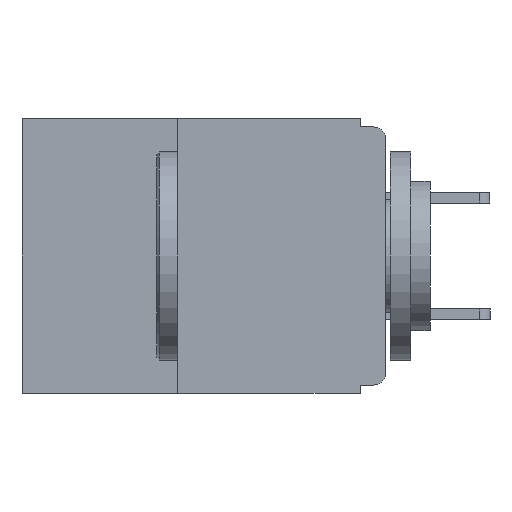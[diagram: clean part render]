
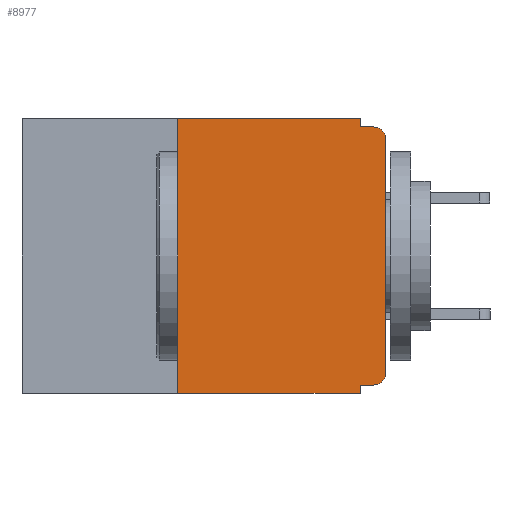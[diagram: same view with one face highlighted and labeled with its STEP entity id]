
A CAD part, left-side view. The second image highlights one B-rep face of the part: STEP entity #8977.
In plain terms, the highlighted planar face has unit normal (-1, 0, 0).
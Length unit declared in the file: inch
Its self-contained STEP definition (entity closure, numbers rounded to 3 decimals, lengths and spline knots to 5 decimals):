
#557 = VERTEX_POINT ( 'NONE', #1101 ) ;
#793 = VERTEX_POINT ( 'NONE', #4445 ) ;
#950 = VERTEX_POINT ( 'NONE', #13284 ) ;
#963 = LINE ( 'NONE', #5021, #13840 ) ;
#1101 = CARTESIAN_POINT ( 'NONE',  ( 0., 0.031, -0.01 ) ) ;
#1429 = EDGE_CURVE ( 'NONE', #14116, #10813, #10999, .T. ) ;
#1709 = ORIENTED_EDGE ( 'NONE', *, *, #15164, .F. ) ;
#1794 = ORIENTED_EDGE ( 'NONE', *, *, #3594, .F. ) ;
#1955 = CARTESIAN_POINT ( 'NONE',  ( 0., 0.015, -0.305 ) ) ;
#2170 = AXIS2_PLACEMENT_3D ( 'NONE', #1955, #12817, #3572 ) ;
#2271 = VERTEX_POINT ( 'NONE', #9158 ) ;
#2395 = ORIENTED_EDGE ( 'NONE', *, *, #1429, .T. ) ;
#2455 = ORIENTED_EDGE ( 'NONE', *, *, #19024, .F. ) ;
#2497 = ORIENTED_EDGE ( 'NONE', *, *, #18966, .F. ) ;
#3142 = LINE ( 'NONE', #9000, #7306 ) ;
#3572 = DIRECTION ( 'NONE',  ( 0., 0., -1. ) ) ;
#3594 = EDGE_CURVE ( 'NONE', #14116, #950, #7839, .T. ) ;
#3626 = CARTESIAN_POINT ( 'NONE',  ( 0., 0.031, -0.33 ) ) ;
#3959 = ORIENTED_EDGE ( 'NONE', *, *, #11931, .T. ) ;
#4445 = CARTESIAN_POINT ( 'NONE',  ( 0., 0., -0.305 ) ) ;
#5021 = CARTESIAN_POINT ( 'NONE',  ( 0., 0.031, 0. ) ) ;
#5065 = CIRCLE ( 'NONE', #2170, 0.015 ) ;
#5336 = DIRECTION ( 'NONE',  ( 0., 0., -1. ) ) ;
#5392 = EDGE_CURVE ( 'NONE', #13097, #19266, #19489, .T. ) ;
#5740 = ORIENTED_EDGE ( 'NONE', *, *, #8612, .T. ) ;
#5884 = DIRECTION ( 'NONE',  ( 0., 1., 0. ) ) ;
#5943 = AXIS2_PLACEMENT_3D ( 'NONE', #12166, #12115, #12102 ) ;
#5947 = DIRECTION ( 'NONE',  ( 0., 0., -1. ) ) ;
#6080 = CARTESIAN_POINT ( 'NONE',  ( 0., 0.25, -0.33 ) ) ;
#6108 = DIRECTION ( 'NONE',  ( 0., 0., 1. ) ) ;
#6459 = PLANE ( 'NONE',  #14403 ) ;
#6658 = VECTOR ( 'NONE', #11596, 39.37008 ) ;
#7191 = CARTESIAN_POINT ( 'NONE',  ( 0., 0.437, 0. ) ) ;
#7194 = DIRECTION ( 'NONE',  ( 0., 0., -1. ) ) ;
#7306 = VECTOR ( 'NONE', #5947, 39.37008 ) ;
#7392 = EDGE_CURVE ( 'NONE', #2271, #557, #963, .T. ) ;
#7514 = DIRECTION ( 'NONE',  ( 1., 0., 0. ) ) ;
#7839 = LINE ( 'NONE', #6080, #8315 ) ;
#8315 = VECTOR ( 'NONE', #6108, 39.37008 ) ;
#8612 = EDGE_CURVE ( 'NONE', #793, #13097, #14703, .T. ) ;
#8803 = VECTOR ( 'NONE', #18542, 39.37008 ) ;
#8830 = CARTESIAN_POINT ( 'NONE',  ( 0., 0., -0.01 ) ) ;
#8956 = VERTEX_POINT ( 'NONE', #16307 ) ;
#8977 = ADVANCED_FACE ( 'NONE', ( #19338 ), #6459, .F. ) ;
#9000 = CARTESIAN_POINT ( 'NONE',  ( 0., 0.031, -0.33 ) ) ;
#9158 = CARTESIAN_POINT ( 'NONE',  ( 0., 0.031, 0. ) ) ;
#9641 = ORIENTED_EDGE ( 'NONE', *, *, #5392, .T. ) ;
#10813 = VERTEX_POINT ( 'NONE', #3626 ) ;
#10845 = ORIENTED_EDGE ( 'NONE', *, *, #15441, .F. ) ;
#10979 = CARTESIAN_POINT ( 'NONE',  ( 0., 0.031, -0.32 ) ) ;
#10999 = LINE ( 'NONE', #18858, #11475 ) ;
#11475 = VECTOR ( 'NONE', #18968, 39.37008 ) ;
#11596 = DIRECTION ( 'NONE',  ( 0., 0., 1. ) ) ;
#11600 = CARTESIAN_POINT ( 'NONE',  ( 0., 0., 0. ) ) ;
#11920 = ORIENTED_EDGE ( 'NONE', *, *, #7392, .F. ) ;
#11931 = EDGE_CURVE ( 'NONE', #8956, #793, #5065, .T. ) ;
#12102 = DIRECTION ( 'NONE',  ( 0., 0., -1. ) ) ;
#12115 = DIRECTION ( 'NONE',  ( -1., 0., 0. ) ) ;
#12153 = LINE ( 'NONE', #8830, #19362 ) ;
#12166 = CARTESIAN_POINT ( 'NONE',  ( 0., 0.015, -0.025 ) ) ;
#12516 = CARTESIAN_POINT ( 'NONE',  ( 0., 0., -0.025 ) ) ;
#12817 = DIRECTION ( 'NONE',  ( -1., 0., 0. ) ) ;
#13097 = VERTEX_POINT ( 'NONE', #12516 ) ;
#13284 = CARTESIAN_POINT ( 'NONE',  ( 0., 0.25, 0. ) ) ;
#13460 = CARTESIAN_POINT ( 'NONE',  ( 0., 0., -0.32 ) ) ;
#13840 = VECTOR ( 'NONE', #5336, 39.37008 ) ;
#13855 = VERTEX_POINT ( 'NONE', #10979 ) ;
#14116 = VERTEX_POINT ( 'NONE', #17583 ) ;
#14239 = CARTESIAN_POINT ( 'NONE',  ( 0., 0.437, 0. ) ) ;
#14403 = AXIS2_PLACEMENT_3D ( 'NONE', #7191, #7514, #7194 ) ;
#14703 = LINE ( 'NONE', #11600, #6658 ) ;
#15164 = EDGE_CURVE ( 'NONE', #950, #2271, #17255, .T. ) ;
#15441 = EDGE_CURVE ( 'NONE', #557, #19266, #12153, .T. ) ;
#16284 = LINE ( 'NONE', #13460, #19507 ) ;
#16307 = CARTESIAN_POINT ( 'NONE',  ( 0., 0.015, -0.32 ) ) ;
#16929 = EDGE_LOOP ( 'NONE', ( #5740, #9641, #10845, #11920, #1709, #1794, #2395, #2455, #2497, #3959 ) ) ;
#17255 = LINE ( 'NONE', #14239, #8803 ) ;
#17583 = CARTESIAN_POINT ( 'NONE',  ( 0., 0.25, -0.33 ) ) ;
#18496 = CARTESIAN_POINT ( 'NONE',  ( 0., 0.015, -0.01 ) ) ;
#18542 = DIRECTION ( 'NONE',  ( 0., -1., 0. ) ) ;
#18858 = CARTESIAN_POINT ( 'NONE',  ( 0., 0.437, -0.33 ) ) ;
#18966 = EDGE_CURVE ( 'NONE', #8956, #13855, #16284, .T. ) ;
#18968 = DIRECTION ( 'NONE',  ( 0., -1., 0. ) ) ;
#19024 = EDGE_CURVE ( 'NONE', #13855, #10813, #3142, .T. ) ;
#19130 = DIRECTION ( 'NONE',  ( 0., -1., 0. ) ) ;
#19266 = VERTEX_POINT ( 'NONE', #18496 ) ;
#19338 = FACE_OUTER_BOUND ( 'NONE', #16929, .T. ) ;
#19362 = VECTOR ( 'NONE', #19130, 39.37008 ) ;
#19489 = CIRCLE ( 'NONE', #5943, 0.015 ) ;
#19507 = VECTOR ( 'NONE', #5884, 39.37008 ) ;
